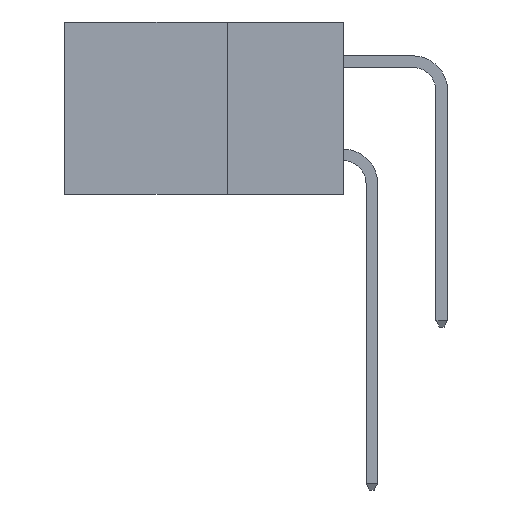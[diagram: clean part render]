
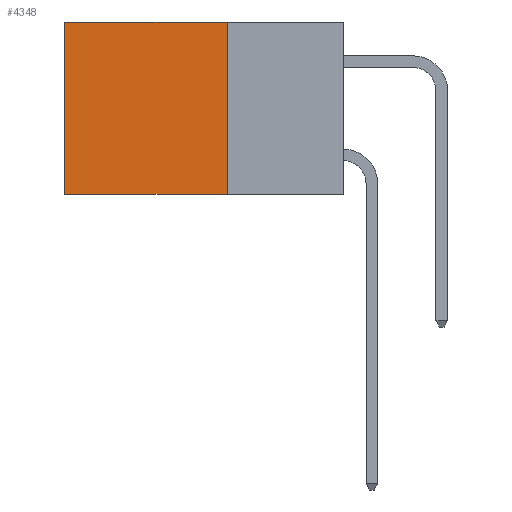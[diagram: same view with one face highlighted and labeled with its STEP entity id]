
A CAD part, left-side view. The second image highlights one B-rep face of the part: STEP entity #4348.
In plain terms, the highlighted planar face has unit normal (-1, 0, 0).
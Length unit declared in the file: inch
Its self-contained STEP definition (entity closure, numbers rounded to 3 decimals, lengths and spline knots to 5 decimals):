
#291 = LINE ( 'NONE', #6705, #3133 ) ;
#723 = LINE ( 'NONE', #3786, #3581 ) ;
#1906 = VECTOR ( 'NONE', #6007, 39.37008 ) ;
#2214 = EDGE_LOOP ( 'NONE', ( #14793, #12356, #15820, #9669 ) ) ;
#3133 = VECTOR ( 'NONE', #5897, 39.37008 ) ;
#3581 = VECTOR ( 'NONE', #3754, 39.37008 ) ;
#3754 = DIRECTION ( 'NONE',  ( 0., 1., 0. ) ) ;
#3786 = CARTESIAN_POINT ( 'NONE',  ( 0.2615, 0.25, -0.37 ) ) ;
#4348 = ADVANCED_FACE ( 'NONE', ( #15541 ), #12070, .F. ) ;
#5534 = VERTEX_POINT ( 'NONE', #13022 ) ;
#5897 = DIRECTION ( 'NONE',  ( 0., 0., -1. ) ) ;
#6007 = DIRECTION ( 'NONE',  ( 0., 0., -1. ) ) ;
#6108 = CARTESIAN_POINT ( 'NONE',  ( 0.2615, 0.6, -0.37 ) ) ;
#6244 = LINE ( 'NONE', #15461, #9186 ) ;
#6347 = VERTEX_POINT ( 'NONE', #13669 ) ;
#6705 = CARTESIAN_POINT ( 'NONE',  ( 0.2615, 0.25, -0.37 ) ) ;
#6861 = EDGE_CURVE ( 'NONE', #7631, #6347, #291, .T. ) ;
#7631 = VERTEX_POINT ( 'NONE', #14995 ) ;
#9186 = VECTOR ( 'NONE', #14220, 39.37008 ) ;
#9669 = ORIENTED_EDGE ( 'NONE', *, *, #13348, .T. ) ;
#11609 = DIRECTION ( 'NONE',  ( 0., 0., -1. ) ) ;
#11759 = EDGE_CURVE ( 'NONE', #6347, #14093, #723, .T. ) ;
#11946 = CARTESIAN_POINT ( 'NONE',  ( 0.2615, 0.25, -0.37 ) ) ;
#12054 = DIRECTION ( 'NONE',  ( 1., 0., 0. ) ) ;
#12070 = PLANE ( 'NONE',  #15076 ) ;
#12356 = ORIENTED_EDGE ( 'NONE', *, *, #11759, .F. ) ;
#13022 = CARTESIAN_POINT ( 'NONE',  ( 0.2615, 0.6, 0. ) ) ;
#13348 = EDGE_CURVE ( 'NONE', #7631, #5534, #6244, .T. ) ;
#13540 = CARTESIAN_POINT ( 'NONE',  ( 0.2615, 0.6, -0.37 ) ) ;
#13669 = CARTESIAN_POINT ( 'NONE',  ( 0.2615, 0.25, -0.37 ) ) ;
#14093 = VERTEX_POINT ( 'NONE', #13540 ) ;
#14220 = DIRECTION ( 'NONE',  ( 0., 1., 0. ) ) ;
#14691 = EDGE_CURVE ( 'NONE', #5534, #14093, #14844, .T. ) ;
#14793 = ORIENTED_EDGE ( 'NONE', *, *, #14691, .T. ) ;
#14844 = LINE ( 'NONE', #6108, #1906 ) ;
#14995 = CARTESIAN_POINT ( 'NONE',  ( 0.2615, 0.25, 0. ) ) ;
#15076 = AXIS2_PLACEMENT_3D ( 'NONE', #11946, #12054, #11609 ) ;
#15461 = CARTESIAN_POINT ( 'NONE',  ( 0.2615, 0.25, 0. ) ) ;
#15541 = FACE_OUTER_BOUND ( 'NONE', #2214, .T. ) ;
#15820 = ORIENTED_EDGE ( 'NONE', *, *, #6861, .F. ) ;
